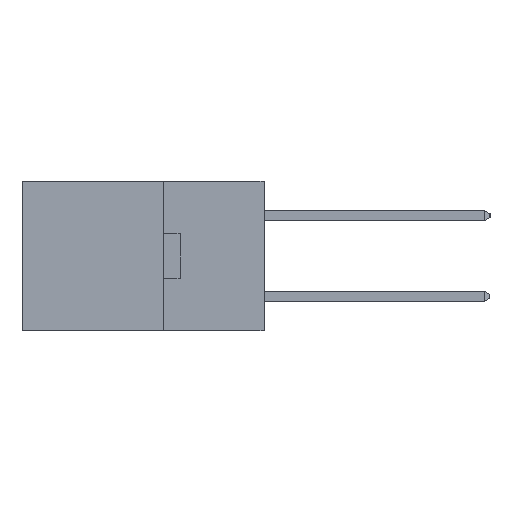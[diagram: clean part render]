
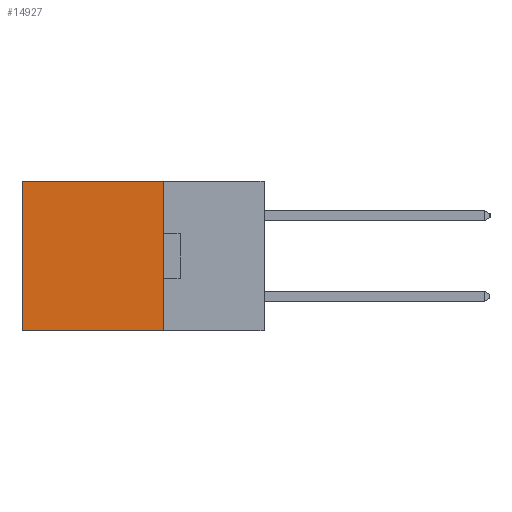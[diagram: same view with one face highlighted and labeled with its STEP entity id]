
A CAD part, left-side view. The second image highlights one B-rep face of the part: STEP entity #14927.
In plain terms, the highlighted planar face has unit normal (-1, 0, 0).
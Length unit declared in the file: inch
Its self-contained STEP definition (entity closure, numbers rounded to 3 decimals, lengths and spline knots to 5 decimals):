
#829 = CARTESIAN_POINT ( 'NONE',  ( 0.2615, 0.25, 0. ) ) ;
#2511 = DIRECTION ( 'NONE',  ( 0., 1., 0. ) ) ;
#2929 = CARTESIAN_POINT ( 'NONE',  ( 0.2615, 0.25, -0.37 ) ) ;
#3074 = VECTOR ( 'NONE', #9557, 39.37008 ) ;
#3566 = VECTOR ( 'NONE', #23197, 39.37008 ) ;
#3744 = PLANE ( 'NONE',  #11771 ) ;
#4391 = VERTEX_POINT ( 'NONE', #17825 ) ;
#6882 = CARTESIAN_POINT ( 'NONE',  ( 0.2615, 0.25, -0.37 ) ) ;
#7398 = ORIENTED_EDGE ( 'NONE', *, *, #14902, .T. ) ;
#7835 = LINE ( 'NONE', #25285, #9897 ) ;
#9557 = DIRECTION ( 'NONE',  ( 0., 1., 0. ) ) ;
#9897 = VECTOR ( 'NONE', #22445, 39.37008 ) ;
#10042 = CARTESIAN_POINT ( 'NONE',  ( 0.2615, 0.25, -0.37 ) ) ;
#10737 = ORIENTED_EDGE ( 'NONE', *, *, #13410, .F. ) ;
#11694 = LINE ( 'NONE', #829, #3074 ) ;
#11771 = AXIS2_PLACEMENT_3D ( 'NONE', #10042, #23333, #12462 ) ;
#11898 = CARTESIAN_POINT ( 'NONE',  ( 0.2615, 0.6, -0.37 ) ) ;
#12462 = DIRECTION ( 'NONE',  ( 0., 0., -1. ) ) ;
#12733 = VERTEX_POINT ( 'NONE', #11898 ) ;
#13410 = EDGE_CURVE ( 'NONE', #20451, #26170, #7835, .T. ) ;
#14641 = LINE ( 'NONE', #23049, #3566 ) ;
#14825 = ORIENTED_EDGE ( 'NONE', *, *, #25692, .F. ) ;
#14902 = EDGE_CURVE ( 'NONE', #4391, #12733, #14641, .T. ) ;
#14927 = ADVANCED_FACE ( 'NONE', ( #20932 ), #3744, .F. ) ;
#15663 = ORIENTED_EDGE ( 'NONE', *, *, #28044, .T. ) ;
#17157 = VECTOR ( 'NONE', #2511, 39.37008 ) ;
#17825 = CARTESIAN_POINT ( 'NONE',  ( 0.2615, 0.6, 0. ) ) ;
#18515 = EDGE_LOOP ( 'NONE', ( #7398, #14825, #10737, #15663 ) ) ;
#18877 = CARTESIAN_POINT ( 'NONE',  ( 0.2615, 0.25, 0. ) ) ;
#20251 = LINE ( 'NONE', #2929, #17157 ) ;
#20451 = VERTEX_POINT ( 'NONE', #18877 ) ;
#20932 = FACE_OUTER_BOUND ( 'NONE', #18515, .T. ) ;
#22445 = DIRECTION ( 'NONE',  ( 0., 0., -1. ) ) ;
#23049 = CARTESIAN_POINT ( 'NONE',  ( 0.2615, 0.6, -0.37 ) ) ;
#23197 = DIRECTION ( 'NONE',  ( 0., 0., -1. ) ) ;
#23333 = DIRECTION ( 'NONE',  ( 1., 0., 0. ) ) ;
#25285 = CARTESIAN_POINT ( 'NONE',  ( 0.2615, 0.25, -0.37 ) ) ;
#25692 = EDGE_CURVE ( 'NONE', #26170, #12733, #20251, .T. ) ;
#26170 = VERTEX_POINT ( 'NONE', #6882 ) ;
#28044 = EDGE_CURVE ( 'NONE', #20451, #4391, #11694, .T. ) ;
